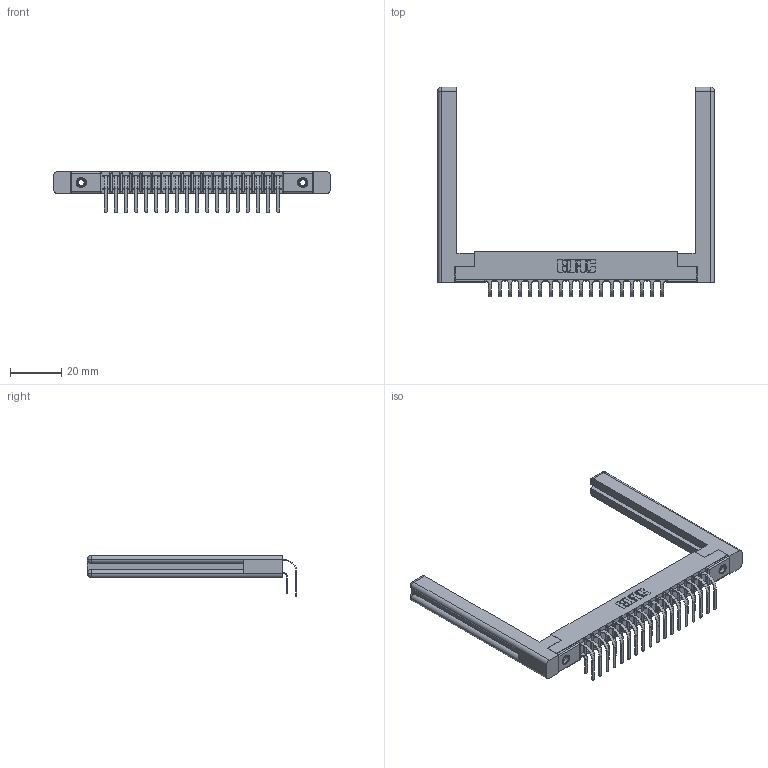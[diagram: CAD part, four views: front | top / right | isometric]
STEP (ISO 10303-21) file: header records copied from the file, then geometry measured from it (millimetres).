
FILE_DESCRIPTION (( 'STEP AP203' ), '1' );
FILE_NAME ('307-036-559-258.STEP', '2022-07-08T16:19:22', ( '' ), ( '' ), 'SwSTEP 2.0', 'SolidWorks 2020', '' );
FILE_SCHEMA (( 'CONFIG_CONTROL_DESIGN' ));
Length unit declared in the file: inch
Products named in the file (6): 307-036-559-258; 307-290-001_558 559 - 1 (Single); 307-220-058; 345-250-001_345-250-001-102; 307-290-001_559 - 2 (Single); 307 Part_.156 Dia Mounting Holes
Assembly tree (41 placements, depth 2):
  307-036-559-258
    307 Part_.156 Dia Mounting Holes
    307-290-001_558 559 - 1 (Single)  x18
    307-290-001_559 - 2 (Single)  x18
    307-220-058  x2
    345-250-001_345-250-001-102  x2
Bounding box: 107.95 x 81.83 x 16.08 mm (x, y, z)
Volume: 14883.6 mm3; surface area: 18345.6 mm2
Topology: 41 solids, 41 shells, 2079 faces, 5789 edges, 3746 vertices
Faces by surface type: plane 1342, cylinder 675, sphere 38, torus 12, cone 12
Entity records: 23046 total; most frequent: CARTESIAN_POINT 3799, ORIENTED_EDGE 3704, DIRECTION 3688, EDGE_CURVE 1852, LINE 1406, VECTOR 1406, VERTEX_POINT 1198, AXIS2_PLACEMENT_3D 1141
